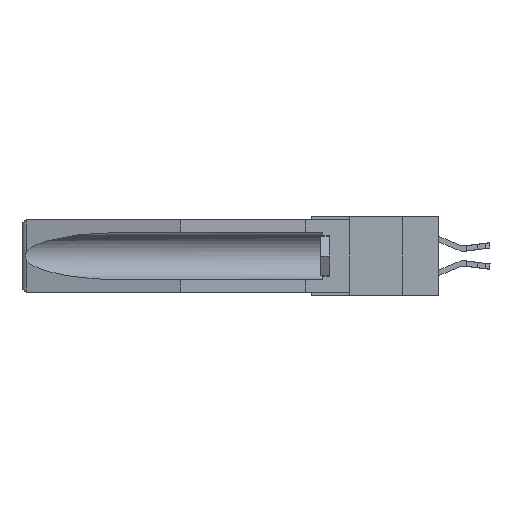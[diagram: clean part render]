
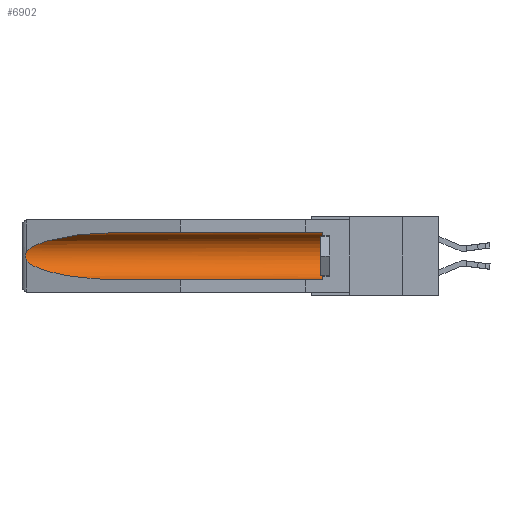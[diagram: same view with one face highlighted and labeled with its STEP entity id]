
A CAD part, left-side view. The second image highlights one B-rep face of the part: STEP entity #6902.
In plain terms, the highlighted cylindrical face has radius 2.857 mm (diameter 5.715 mm), a partial arc.
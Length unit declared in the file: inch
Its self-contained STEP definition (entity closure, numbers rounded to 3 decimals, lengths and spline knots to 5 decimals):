
#371 = CARTESIAN_POINT ( 'NONE',  ( 0.2675, 1.53308, -0.17534 ) ) ;
#1014 = EDGE_CURVE ( 'NONE', #14479, #10723, #25229, .T. ) ;
#1291 = DIRECTION ( 'NONE',  ( 0., 1., 0. ) ) ;
#2080 =( BOUNDED_CURVE ( )  B_SPLINE_CURVE ( 3, ( #17068, #14351, #23871, #7744 ),
 .UNSPECIFIED., .F., .F. ) 
 B_SPLINE_CURVE_WITH_KNOTS ( ( 4, 4 ),
 ( 4.71239, 6.08839 ),
 .UNSPECIFIED. ) 
 CURVE ( )  GEOMETRIC_REPRESENTATION_ITEM ( )  RATIONAL_B_SPLINE_CURVE ( ( 1., 0.848, 0.848, 1. ) ) 
 REPRESENTATION_ITEM ( '' )  );
#2804 = CARTESIAN_POINT ( 'NONE',  ( 0.26537, 1.52718, -0.14972 ) ) ;
#2919 = ORIENTED_EDGE ( 'NONE', *, *, #12286, .T. ) ;
#3007 = CARTESIAN_POINT ( 'NONE',  ( 0.26654, 1.53092, -0.15636 ) ) ;
#3126 = ORIENTED_EDGE ( 'NONE', *, *, #1014, .T. ) ;
#3241 = CARTESIAN_POINT ( 'NONE',  ( 0.26537, 1.52718, -0.19328 ) ) ;
#3437 = EDGE_CURVE ( 'NONE', #14479, #25042, #5677, .T. ) ;
#3613 = AXIS2_PLACEMENT_3D ( 'NONE', #19787, #17507, #28955 ) ;
#4040 = CARTESIAN_POINT ( 'NONE',  ( 0.26537, 1.52718, -0.19328 ) ) ;
#5192 = CARTESIAN_POINT ( 'NONE',  ( 0.26655, 1.53094, -0.18657 ) ) ;
#5623 = EDGE_LOOP ( 'NONE', ( #7449, #17455, #14242, #23251, #3126, #2919 ) ) ;
#5677 = LINE ( 'NONE', #28016, #22211 ) ;
#6902 = ADVANCED_FACE ( 'NONE', ( #18106 ), #24915, .F. ) ;
#7449 = ORIENTED_EDGE ( 'NONE', *, *, #10403, .T. ) ;
#7497 = CARTESIAN_POINT ( 'NONE',  ( 0.2673, 1.53269, -0.17917 ) ) ;
#7598 = CARTESIAN_POINT ( 'NONE',  ( 0.26537, 1.52718, -0.19328 ) ) ;
#7737 = CARTESIAN_POINT ( 'NONE',  ( 0.155, 1.07973, -0.284 ) ) ;
#7744 = CARTESIAN_POINT ( 'NONE',  ( 0.26537, 1.52718, -0.14972 ) ) ;
#7832 = LINE ( 'NONE', #21515, #22228 ) ;
#9296 = EDGE_CURVE ( 'NONE', #25172, #25042, #11429, .T. ) ;
#9593 = CARTESIAN_POINT ( 'NONE',  ( 0.26597, 1.52961, -0.15275 ) ) ;
#10403 = EDGE_CURVE ( 'NONE', #24137, #25750, #2080, .T. ) ;
#10723 = VERTEX_POINT ( 'NONE', #16923 ) ;
#11129 = DIRECTION ( 'NONE',  ( 0., 1., 0. ) ) ;
#11429 =( BOUNDED_CURVE ( )  B_SPLINE_CURVE ( 3, ( #3241, #17064, #26385, #7737 ),
 .UNSPECIFIED., .F., .F. ) 
 B_SPLINE_CURVE_WITH_KNOTS ( ( 4, 4 ),
 ( 0.1948, 1.5708 ),
 .UNSPECIFIED. ) 
 CURVE ( )  GEOMETRIC_REPRESENTATION_ITEM ( )  RATIONAL_B_SPLINE_CURVE ( ( 1., 0.848, 0.848, 1. ) ) 
 REPRESENTATION_ITEM ( '' )  );
#12286 = EDGE_CURVE ( 'NONE', #10723, #24137, #7832, .T. ) ;
#13162 = CARTESIAN_POINT ( 'NONE',  ( 0.155, 1.07973, -0.284 ) ) ;
#13525 = DIRECTION ( 'NONE',  ( 0., 0., 1. ) ) ;
#14242 = ORIENTED_EDGE ( 'NONE', *, *, #9296, .T. ) ;
#14305 = CARTESIAN_POINT ( 'NONE',  ( 0.2675, 1.53308, -0.16763 ) ) ;
#14351 = CARTESIAN_POINT ( 'NONE',  ( 0.21114, 1.30732, -0.059 ) ) ;
#14479 = VERTEX_POINT ( 'NONE', #27306 ) ;
#14528 = DIRECTION ( 'NONE',  ( 0., 1., 0. ) ) ;
#15992 = AXIS2_PLACEMENT_3D ( 'NONE', #29329, #11129, #13525 ) ;
#16923 = CARTESIAN_POINT ( 'NONE',  ( 0.155, 0.126, -0.059 ) ) ;
#17064 = CARTESIAN_POINT ( 'NONE',  ( 0.25451, 1.48313, -0.24835 ) ) ;
#17068 = CARTESIAN_POINT ( 'NONE',  ( 0.155, 1.07973, -0.059 ) ) ;
#17455 = ORIENTED_EDGE ( 'NONE', *, *, #28564, .T. ) ;
#17507 = DIRECTION ( 'NONE',  ( 0., -1., 0. ) ) ;
#18095 = CARTESIAN_POINT ( 'NONE',  ( 0.26537, 1.52718, -0.14972 ) ) ;
#18106 = FACE_OUTER_BOUND ( 'NONE', #5623, .T. ) ;
#19016 = CARTESIAN_POINT ( 'NONE',  ( 0.26597, 1.5296, -0.19026 ) ) ;
#19787 = CARTESIAN_POINT ( 'NONE',  ( 0.155, 0.126, -0.1715 ) ) ;
#21515 = CARTESIAN_POINT ( 'NONE',  ( 0.155, -0.30754, -0.059 ) ) ;
#22056 = CARTESIAN_POINT ( 'NONE',  ( 0.155, 1.07973, -0.059 ) ) ;
#22211 = VECTOR ( 'NONE', #14528, 39.37008 ) ;
#22228 = VECTOR ( 'NONE', #1291, 39.37008 ) ;
#23251 = ORIENTED_EDGE ( 'NONE', *, *, #3437, .F. ) ;
#23871 = CARTESIAN_POINT ( 'NONE',  ( 0.25451, 1.48313, -0.09465 ) ) ;
#24137 = VERTEX_POINT ( 'NONE', #22056 ) ;
#24915 = CYLINDRICAL_SURFACE ( 'NONE', #15992, 0.1125 ) ;
#25042 = VERTEX_POINT ( 'NONE', #13162 ) ;
#25172 = VERTEX_POINT ( 'NONE', #4040 ) ;
#25229 = CIRCLE ( 'NONE', #3613, 0.1125 ) ;
#25750 = VERTEX_POINT ( 'NONE', #18095 ) ;
#26385 = CARTESIAN_POINT ( 'NONE',  ( 0.21114, 1.30732, -0.284 ) ) ;
#27033 = B_SPLINE_CURVE_WITH_KNOTS ( 'NONE', 3,
 ( #2804, #9593, #3007, #27904, #14305, #371, #7497, #5192, #19016, #7598 ),
 .UNSPECIFIED., .F., .F.,
 ( 4, 2, 2, 2, 4 ),
 ( 0., 0.00029, 0.00058, 0.00087, 0.00117 ),
 .UNSPECIFIED. ) ;
#27306 = CARTESIAN_POINT ( 'NONE',  ( 0.155, 0.126, -0.284 ) ) ;
#27904 = CARTESIAN_POINT ( 'NONE',  ( 0.2673, 1.5327, -0.16383 ) ) ;
#28016 = CARTESIAN_POINT ( 'NONE',  ( 0.155, -0.30754, -0.284 ) ) ;
#28564 = EDGE_CURVE ( 'NONE', #25750, #25172, #27033, .T. ) ;
#28955 = DIRECTION ( 'NONE',  ( 0., 0., 1. ) ) ;
#29329 = CARTESIAN_POINT ( 'NONE',  ( 0.155, -0.30754, -0.1715 ) ) ;
